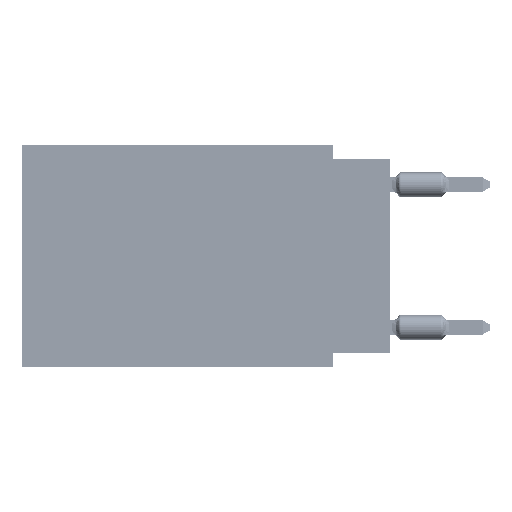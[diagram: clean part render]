
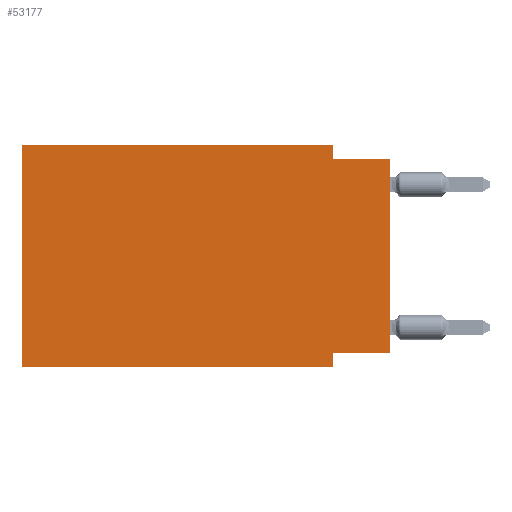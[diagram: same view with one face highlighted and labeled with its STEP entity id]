
A CAD part, left-side view. The second image highlights one B-rep face of the part: STEP entity #53177.
In plain terms, the highlighted planar face has unit normal (-1, 0, 0).
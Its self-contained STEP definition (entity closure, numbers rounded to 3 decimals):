
#101 = ORIENTED_EDGE ( 'NONE', *, *, #8972, .F. ) ;
#643 = VECTOR ( 'NONE', #55705, 1000. ) ;
#790 = DIRECTION ( 'NONE',  ( 0., -1., 0. ) ) ;
#1089 = VECTOR ( 'NONE', #55524, 1000. ) ;
#1540 = LINE ( 'NONE', #5536, #22453 ) ;
#3097 = VECTOR ( 'NONE', #790, 1000. ) ;
#3396 = DIRECTION ( 'NONE',  ( 0., 0., -1. ) ) ;
#4901 = DIRECTION ( 'NONE',  ( 0., -1., 0. ) ) ;
#5536 = CARTESIAN_POINT ( 'NONE',  ( 0., 0., -9.271 ) ) ;
#5568 = CARTESIAN_POINT ( 'NONE',  ( 0., 2.54, 0. ) ) ;
#5760 = ORIENTED_EDGE ( 'NONE', *, *, #51615, .F. ) ;
#8922 = VECTOR ( 'NONE', #52852, 1000. ) ;
#8972 = EDGE_CURVE ( 'NONE', #12541, #36278, #43268, .T. ) ;
#10336 = DIRECTION ( 'NONE',  ( 0., 0., 1. ) ) ;
#11118 = VERTEX_POINT ( 'NONE', #25935 ) ;
#11338 = CARTESIAN_POINT ( 'NONE',  ( 0., 16.383, -9.906 ) ) ;
#12541 = VERTEX_POINT ( 'NONE', #31348 ) ;
#14621 = LINE ( 'NONE', #23755, #25319 ) ;
#16435 = AXIS2_PLACEMENT_3D ( 'NONE', #56071, #29977, #3396 ) ;
#18021 = VERTEX_POINT ( 'NONE', #41096 ) ;
#18939 = DIRECTION ( 'NONE',  ( 0., 1., 0. ) ) ;
#20147 = EDGE_CURVE ( 'NONE', #42899, #11118, #46353, .T. ) ;
#20828 = CARTESIAN_POINT ( 'NONE',  ( 0., 16.383, -9.906 ) ) ;
#21496 = ORIENTED_EDGE ( 'NONE', *, *, #45774, .F. ) ;
#22453 = VECTOR ( 'NONE', #18939, 1000. ) ;
#23755 = CARTESIAN_POINT ( 'NONE',  ( 0., 16.383, 0. ) ) ;
#24464 = EDGE_LOOP ( 'NONE', ( #45923, #21496, #50965, #101, #5760, #42417, #33777, #34422 ) ) ;
#25309 = CARTESIAN_POINT ( 'NONE',  ( 0., 0., 0. ) ) ;
#25319 = VECTOR ( 'NONE', #10336, 1000. ) ;
#25935 = CARTESIAN_POINT ( 'NONE',  ( 0., 2.54, -9.906 ) ) ;
#29977 = DIRECTION ( 'NONE',  ( 1., 0., 0. ) ) ;
#31313 = LINE ( 'NONE', #5568, #8922 ) ;
#31348 = CARTESIAN_POINT ( 'NONE',  ( 0., 16.383, 0. ) ) ;
#31701 = EDGE_CURVE ( 'NONE', #34356, #51932, #1540, .T. ) ;
#32065 = VECTOR ( 'NONE', #4901, 1000. ) ;
#33230 = CARTESIAN_POINT ( 'NONE',  ( 0., 0., -9.271 ) ) ;
#33345 = DIRECTION ( 'NONE',  ( 0., 0., 1. ) ) ;
#33633 = LINE ( 'NONE', #38232, #643 ) ;
#33725 = EDGE_CURVE ( 'NONE', #36278, #53513, #31313, .T. ) ;
#33777 = ORIENTED_EDGE ( 'NONE', *, *, #51394, .F. ) ;
#34356 = VERTEX_POINT ( 'NONE', #33230 ) ;
#34422 = ORIENTED_EDGE ( 'NONE', *, *, #31701, .F. ) ;
#35403 = CARTESIAN_POINT ( 'NONE',  ( 0., 0., -0.635 ) ) ;
#36278 = VERTEX_POINT ( 'NONE', #56591 ) ;
#37735 = VECTOR ( 'NONE', #33345, 1000. ) ;
#38232 = CARTESIAN_POINT ( 'NONE',  ( 0., 2.54, -9.906 ) ) ;
#38298 = CARTESIAN_POINT ( 'NONE',  ( 0., 2.54, -9.271 ) ) ;
#41096 = CARTESIAN_POINT ( 'NONE',  ( 0., 0., -0.635 ) ) ;
#42417 = ORIENTED_EDGE ( 'NONE', *, *, #20147, .T. ) ;
#42889 = FACE_OUTER_BOUND ( 'NONE', #24464, .T. ) ;
#42899 = VERTEX_POINT ( 'NONE', #11338 ) ;
#43169 = PLANE ( 'NONE',  #16435 ) ;
#43268 = LINE ( 'NONE', #44108, #32065 ) ;
#44108 = CARTESIAN_POINT ( 'NONE',  ( 0., 16.383, 0. ) ) ;
#44777 = EDGE_CURVE ( 'NONE', #34356, #18021, #54862, .T. ) ;
#45774 = EDGE_CURVE ( 'NONE', #53513, #18021, #52637, .T. ) ;
#45923 = ORIENTED_EDGE ( 'NONE', *, *, #44777, .T. ) ;
#46353 = LINE ( 'NONE', #20828, #1089 ) ;
#46550 = CARTESIAN_POINT ( 'NONE',  ( 0., 2.54, -0.635 ) ) ;
#50965 = ORIENTED_EDGE ( 'NONE', *, *, #33725, .F. ) ;
#51394 = EDGE_CURVE ( 'NONE', #51932, #11118, #33633, .T. ) ;
#51615 = EDGE_CURVE ( 'NONE', #42899, #12541, #14621, .T. ) ;
#51932 = VERTEX_POINT ( 'NONE', #38298 ) ;
#52637 = LINE ( 'NONE', #35403, #3097 ) ;
#52852 = DIRECTION ( 'NONE',  ( 0., 0., -1. ) ) ;
#53177 = ADVANCED_FACE ( 'NONE', ( #42889 ), #43169, .F. ) ;
#53513 = VERTEX_POINT ( 'NONE', #46550 ) ;
#54862 = LINE ( 'NONE', #25309, #37735 ) ;
#55524 = DIRECTION ( 'NONE',  ( 0., -1., 0. ) ) ;
#55705 = DIRECTION ( 'NONE',  ( 0., 0., -1. ) ) ;
#56071 = CARTESIAN_POINT ( 'NONE',  ( 0., 16.383, 0. ) ) ;
#56591 = CARTESIAN_POINT ( 'NONE',  ( 0., 2.54, 0. ) ) ;
